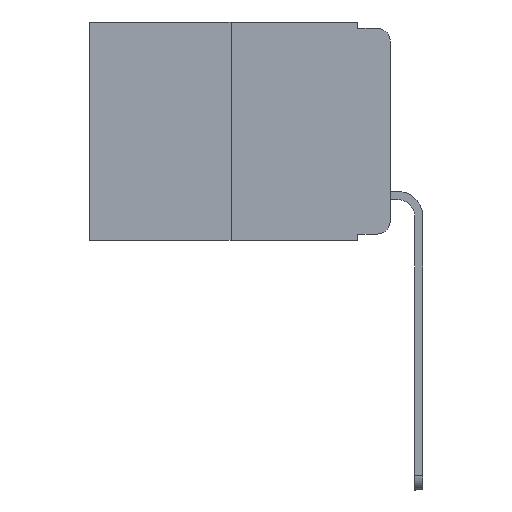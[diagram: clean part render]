
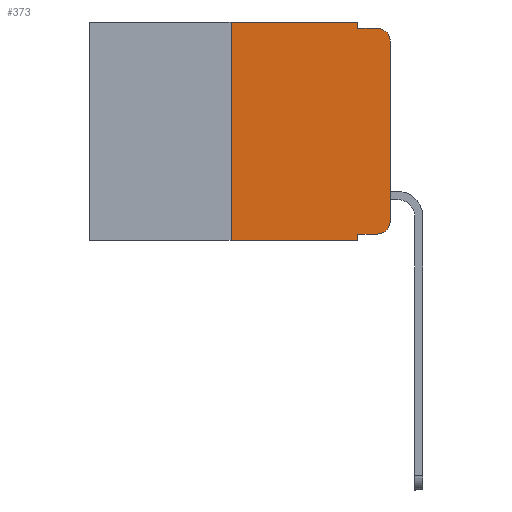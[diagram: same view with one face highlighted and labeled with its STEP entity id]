
A CAD part, left-side view. The second image highlights one B-rep face of the part: STEP entity #373.
In plain terms, the highlighted planar face has unit normal (-1, 0, 0).
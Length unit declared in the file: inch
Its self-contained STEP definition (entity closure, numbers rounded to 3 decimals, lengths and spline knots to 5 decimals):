
#206 = EDGE_CURVE ( 'NONE', #11889, #3587, #6726, .T. ) ;
#373 = ADVANCED_FACE ( 'NONE', ( #6857 ), #4295, .F. ) ;
#409 = VECTOR ( 'NONE', #5190, 39.37008 ) ;
#437 = CARTESIAN_POINT ( 'NONE',  ( 0., 0.051, -0.333 ) ) ;
#609 = CARTESIAN_POINT ( 'NONE',  ( 0., 0.051, -0.01 ) ) ;
#697 = CARTESIAN_POINT ( 'NONE',  ( 0., 0.051, 0. ) ) ;
#934 = DIRECTION ( 'NONE',  ( 0., 0., 1. ) ) ;
#1436 = EDGE_CURVE ( 'NONE', #5542, #11356, #8648, .T. ) ;
#1731 = DIRECTION ( 'NONE',  ( 0., -1., 0. ) ) ;
#1888 = CARTESIAN_POINT ( 'NONE',  ( 0., 0., -0.03 ) ) ;
#2079 = LINE ( 'NONE', #6162, #10999 ) ;
#2470 = CARTESIAN_POINT ( 'NONE',  ( 0., 0.25, 0. ) ) ;
#2500 = EDGE_CURVE ( 'NONE', #7750, #9712, #9318, .T. ) ;
#2692 = DIRECTION ( 'NONE',  ( 0., 0., -1. ) ) ;
#2876 = DIRECTION ( 'NONE',  ( 0., 0., -1. ) ) ;
#3228 = CARTESIAN_POINT ( 'NONE',  ( 0., 0.473, -0.343 ) ) ;
#3471 = VERTEX_POINT ( 'NONE', #4865 ) ;
#3513 = EDGE_CURVE ( 'NONE', #10820, #11889, #8988, .T. ) ;
#3587 = VERTEX_POINT ( 'NONE', #4134 ) ;
#3695 = VECTOR ( 'NONE', #2876, 39.37008 ) ;
#3795 = CARTESIAN_POINT ( 'NONE',  ( 0., 0.051, -0.333 ) ) ;
#3922 = VERTEX_POINT ( 'NONE', #12101 ) ;
#4094 = LINE ( 'NONE', #3228, #7274 ) ;
#4119 = CARTESIAN_POINT ( 'NONE',  ( 0., 0.051, 0. ) ) ;
#4134 = CARTESIAN_POINT ( 'NONE',  ( 0., 0.02, -0.01 ) ) ;
#4295 = PLANE ( 'NONE',  #11896 ) ;
#4532 = DIRECTION ( 'NONE',  ( 0., 0., 1. ) ) ;
#4800 = VECTOR ( 'NONE', #1731, 39.37008 ) ;
#4865 = CARTESIAN_POINT ( 'NONE',  ( 0., 0., -0.313 ) ) ;
#4992 = CARTESIAN_POINT ( 'NONE',  ( 0., 0.473, 0. ) ) ;
#5190 = DIRECTION ( 'NONE',  ( 0., 0., -1. ) ) ;
#5373 = VECTOR ( 'NONE', #5385, 39.37008 ) ;
#5385 = DIRECTION ( 'NONE',  ( 0., -1., 0. ) ) ;
#5542 = VERTEX_POINT ( 'NONE', #11559 ) ;
#5832 = CARTESIAN_POINT ( 'NONE',  ( 0., 0.25, 0. ) ) ;
#5854 = ORIENTED_EDGE ( 'NONE', *, *, #12216, .T. ) ;
#5867 = ORIENTED_EDGE ( 'NONE', *, *, #2500, .F. ) ;
#5939 = ORIENTED_EDGE ( 'NONE', *, *, #11878, .F. ) ;
#5981 = DIRECTION ( 'NONE',  ( 0., 0., -1. ) ) ;
#6162 = CARTESIAN_POINT ( 'NONE',  ( 0., 0., 0. ) ) ;
#6242 = CARTESIAN_POINT ( 'NONE',  ( 0., 0.473, 0. ) ) ;
#6254 = VECTOR ( 'NONE', #10886, 39.37008 ) ;
#6386 = DIRECTION ( 'NONE',  ( 0., -1., 0. ) ) ;
#6394 = ORIENTED_EDGE ( 'NONE', *, *, #6419, .T. ) ;
#6419 = EDGE_CURVE ( 'NONE', #3922, #3471, #6747, .T. ) ;
#6581 = EDGE_CURVE ( 'NONE', #7750, #3922, #10800, .T. ) ;
#6726 = LINE ( 'NONE', #609, #6254 ) ;
#6747 = CIRCLE ( 'NONE', #11101, 0.02 ) ;
#6856 = ORIENTED_EDGE ( 'NONE', *, *, #12811, .T. ) ;
#6857 = FACE_OUTER_BOUND ( 'NONE', #10002, .T. ) ;
#7247 = DIRECTION ( 'NONE',  ( 1., 0., 0. ) ) ;
#7274 = VECTOR ( 'NONE', #6386, 39.37008 ) ;
#7715 = AXIS2_PLACEMENT_3D ( 'NONE', #8815, #11956, #2692 ) ;
#7750 = VERTEX_POINT ( 'NONE', #437 ) ;
#8648 = LINE ( 'NONE', #2470, #12668 ) ;
#8678 = ORIENTED_EDGE ( 'NONE', *, *, #12330, .T. ) ;
#8815 = CARTESIAN_POINT ( 'NONE',  ( 0., 0.02, -0.03 ) ) ;
#8927 = CARTESIAN_POINT ( 'NONE',  ( 0., 0.051, 0. ) ) ;
#8988 = LINE ( 'NONE', #8927, #3695 ) ;
#9318 = LINE ( 'NONE', #4119, #409 ) ;
#9712 = VERTEX_POINT ( 'NONE', #12560 ) ;
#10002 = EDGE_LOOP ( 'NONE', ( #6856, #5854, #10358, #12590, #5939, #13224, #8678, #5867, #13006, #6394 ) ) ;
#10163 = LINE ( 'NONE', #4992, #5373 ) ;
#10358 = ORIENTED_EDGE ( 'NONE', *, *, #206, .F. ) ;
#10558 = CIRCLE ( 'NONE', #7715, 0.02 ) ;
#10800 = LINE ( 'NONE', #3795, #4800 ) ;
#10820 = VERTEX_POINT ( 'NONE', #697 ) ;
#10886 = DIRECTION ( 'NONE',  ( 0., -1., 0. ) ) ;
#10957 = CARTESIAN_POINT ( 'NONE',  ( 0., 0.02, -0.313 ) ) ;
#10999 = VECTOR ( 'NONE', #934, 39.37008 ) ;
#11101 = AXIS2_PLACEMENT_3D ( 'NONE', #10957, #12096, #5981 ) ;
#11261 = CARTESIAN_POINT ( 'NONE',  ( 0., 0.051, -0.01 ) ) ;
#11356 = VERTEX_POINT ( 'NONE', #5832 ) ;
#11365 = VERTEX_POINT ( 'NONE', #1888 ) ;
#11413 = DIRECTION ( 'NONE',  ( 0., 0., -1. ) ) ;
#11559 = CARTESIAN_POINT ( 'NONE',  ( 0., 0.25, -0.343 ) ) ;
#11878 = EDGE_CURVE ( 'NONE', #11356, #10820, #10163, .T. ) ;
#11889 = VERTEX_POINT ( 'NONE', #11261 ) ;
#11896 = AXIS2_PLACEMENT_3D ( 'NONE', #6242, #7247, #11413 ) ;
#11956 = DIRECTION ( 'NONE',  ( -1., 0., 0. ) ) ;
#12096 = DIRECTION ( 'NONE',  ( -1., 0., 0. ) ) ;
#12101 = CARTESIAN_POINT ( 'NONE',  ( 0., 0.02, -0.333 ) ) ;
#12216 = EDGE_CURVE ( 'NONE', #11365, #3587, #10558, .T. ) ;
#12330 = EDGE_CURVE ( 'NONE', #5542, #9712, #4094, .T. ) ;
#12560 = CARTESIAN_POINT ( 'NONE',  ( 0., 0.051, -0.343 ) ) ;
#12590 = ORIENTED_EDGE ( 'NONE', *, *, #3513, .F. ) ;
#12668 = VECTOR ( 'NONE', #4532, 39.37008 ) ;
#12811 = EDGE_CURVE ( 'NONE', #3471, #11365, #2079, .T. ) ;
#13006 = ORIENTED_EDGE ( 'NONE', *, *, #6581, .T. ) ;
#13224 = ORIENTED_EDGE ( 'NONE', *, *, #1436, .F. ) ;
